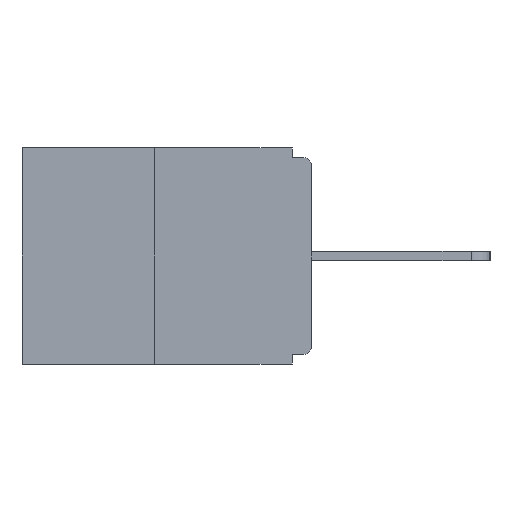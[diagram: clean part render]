
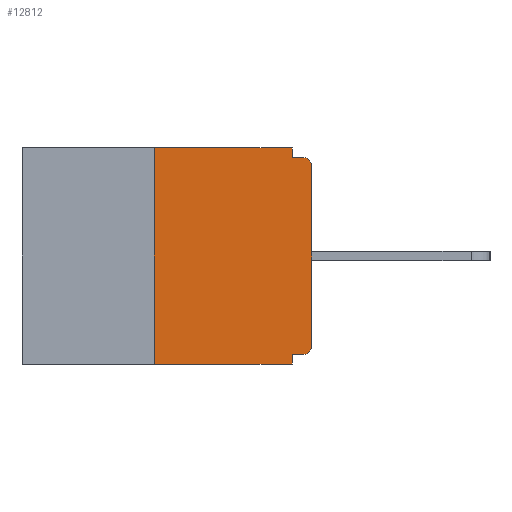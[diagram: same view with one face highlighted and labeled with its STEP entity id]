
A CAD part, left-side view. The second image highlights one B-rep face of the part: STEP entity #12812.
In plain terms, the highlighted planar face has unit normal (-1, 0, 0).
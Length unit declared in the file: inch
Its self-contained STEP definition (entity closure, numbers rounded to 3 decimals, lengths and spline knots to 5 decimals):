
#815 = CARTESIAN_POINT ( 'NONE',  ( 0., 0.015, -0.328 ) ) ;
#1198 = DIRECTION ( 'NONE',  ( 0., -1., 0. ) ) ;
#1641 = ORIENTED_EDGE ( 'NONE', *, *, #5648, .T. ) ;
#1851 = CARTESIAN_POINT ( 'NONE',  ( 0., 0.031, -0.328 ) ) ;
#2156 = CARTESIAN_POINT ( 'NONE',  ( 0., 0.25, -0.343 ) ) ;
#2439 = EDGE_LOOP ( 'NONE', ( #5505, #18324, #3972, #24910, #10209, #16772, #1641, #25115, #24776, #17463 ) ) ;
#2748 = VECTOR ( 'NONE', #23778, 39.37008 ) ;
#2814 = VERTEX_POINT ( 'NONE', #15146 ) ;
#2869 = CARTESIAN_POINT ( 'NONE',  ( 0., 0., -0.328 ) ) ;
#3316 = VECTOR ( 'NONE', #11759, 39.37008 ) ;
#3339 = DIRECTION ( 'NONE',  ( -1., 0., 0. ) ) ;
#3678 = AXIS2_PLACEMENT_3D ( 'NONE', #8820, #10789, #18756 ) ;
#3972 = ORIENTED_EDGE ( 'NONE', *, *, #20627, .T. ) ;
#4026 = CARTESIAN_POINT ( 'NONE',  ( 0., 0.015, -0.015 ) ) ;
#4176 = VERTEX_POINT ( 'NONE', #815 ) ;
#4190 = EDGE_CURVE ( 'NONE', #11388, #22368, #18947, .T. ) ;
#4318 = CIRCLE ( 'NONE', #24548, 0.015 ) ;
#4536 = CARTESIAN_POINT ( 'NONE',  ( 0., 0., -0.03 ) ) ;
#4954 = CARTESIAN_POINT ( 'NONE',  ( 0., 0.25, 0. ) ) ;
#4955 = DIRECTION ( 'NONE',  ( 0., 0., -1. ) ) ;
#5152 = EDGE_CURVE ( 'NONE', #19317, #2814, #7608, .T. ) ;
#5505 = ORIENTED_EDGE ( 'NONE', *, *, #8777, .F. ) ;
#5648 = EDGE_CURVE ( 'NONE', #12283, #21295, #25003, .T. ) ;
#5665 = CARTESIAN_POINT ( 'NONE',  ( 0., 0.25, 0. ) ) ;
#6247 = CIRCLE ( 'NONE', #14596, 0.015 ) ;
#6942 = CARTESIAN_POINT ( 'NONE',  ( 0., 0.031, 0. ) ) ;
#7402 = CARTESIAN_POINT ( 'NONE',  ( 0., 0., -0.313 ) ) ;
#7410 = FACE_OUTER_BOUND ( 'NONE', #2439, .T. ) ;
#7608 = LINE ( 'NONE', #16184, #17377 ) ;
#7834 = EDGE_CURVE ( 'NONE', #21295, #24124, #4318, .T. ) ;
#7877 = CARTESIAN_POINT ( 'NONE',  ( 0., 0., -0.015 ) ) ;
#7922 = VECTOR ( 'NONE', #10638, 39.37008 ) ;
#8051 = CARTESIAN_POINT ( 'NONE',  ( 0., 0., 0. ) ) ;
#8095 = LINE ( 'NONE', #2869, #19121 ) ;
#8693 = VECTOR ( 'NONE', #1198, 39.37008 ) ;
#8777 = EDGE_CURVE ( 'NONE', #22368, #16342, #20468, .T. ) ;
#8820 = CARTESIAN_POINT ( 'NONE',  ( 0., 0.46, 0. ) ) ;
#9101 = CARTESIAN_POINT ( 'NONE',  ( 0., 0.015, -0.03 ) ) ;
#10209 = ORIENTED_EDGE ( 'NONE', *, *, #14150, .F. ) ;
#10638 = DIRECTION ( 'NONE',  ( 0., 0., 1. ) ) ;
#10789 = DIRECTION ( 'NONE',  ( 1., 0., 0. ) ) ;
#10865 = DIRECTION ( 'NONE',  ( 0., 0., -1. ) ) ;
#11388 = VERTEX_POINT ( 'NONE', #2156 ) ;
#11759 = DIRECTION ( 'NONE',  ( 0., -1., 0. ) ) ;
#12283 = VERTEX_POINT ( 'NONE', #7402 ) ;
#12812 = ADVANCED_FACE ( 'NONE', ( #7410 ), #14660, .F. ) ;
#12859 = CARTESIAN_POINT ( 'NONE',  ( 0., 0.46, -0.343 ) ) ;
#13325 = LINE ( 'NONE', #12859, #8693 ) ;
#14150 = EDGE_CURVE ( 'NONE', #4176, #19317, #8095, .T. ) ;
#14414 = DIRECTION ( 'NONE',  ( 0., 0., -1. ) ) ;
#14596 = AXIS2_PLACEMENT_3D ( 'NONE', #22462, #16626, #4955 ) ;
#14660 = PLANE ( 'NONE',  #3678 ) ;
#14987 = VERTEX_POINT ( 'NONE', #17638 ) ;
#15146 = CARTESIAN_POINT ( 'NONE',  ( 0., 0.031, -0.343 ) ) ;
#16184 = CARTESIAN_POINT ( 'NONE',  ( 0., 0.031, -0.343 ) ) ;
#16342 = VERTEX_POINT ( 'NONE', #21648 ) ;
#16626 = DIRECTION ( 'NONE',  ( -1., 0., 0. ) ) ;
#16772 = ORIENTED_EDGE ( 'NONE', *, *, #21399, .T. ) ;
#17377 = VECTOR ( 'NONE', #14414, 39.37008 ) ;
#17463 = ORIENTED_EDGE ( 'NONE', *, *, #19082, .F. ) ;
#17638 = CARTESIAN_POINT ( 'NONE',  ( 0., 0.031, -0.015 ) ) ;
#18324 = ORIENTED_EDGE ( 'NONE', *, *, #4190, .F. ) ;
#18546 = CARTESIAN_POINT ( 'NONE',  ( 0., 0.46, 0. ) ) ;
#18629 = DIRECTION ( 'NONE',  ( 0., -1., 0. ) ) ;
#18756 = DIRECTION ( 'NONE',  ( 0., 0., -1. ) ) ;
#18947 = LINE ( 'NONE', #4954, #7922 ) ;
#19082 = EDGE_CURVE ( 'NONE', #16342, #14987, #19518, .T. ) ;
#19121 = VECTOR ( 'NONE', #20424, 39.37008 ) ;
#19194 = VECTOR ( 'NONE', #10865, 39.37008 ) ;
#19317 = VERTEX_POINT ( 'NONE', #1851 ) ;
#19518 = LINE ( 'NONE', #6942, #19194 ) ;
#20187 = VECTOR ( 'NONE', #18629, 39.37008 ) ;
#20424 = DIRECTION ( 'NONE',  ( 0., 1., 0. ) ) ;
#20468 = LINE ( 'NONE', #18546, #20187 ) ;
#20627 = EDGE_CURVE ( 'NONE', #11388, #2814, #13325, .T. ) ;
#21295 = VERTEX_POINT ( 'NONE', #4536 ) ;
#21399 = EDGE_CURVE ( 'NONE', #4176, #12283, #6247, .T. ) ;
#21648 = CARTESIAN_POINT ( 'NONE',  ( 0., 0.031, 0. ) ) ;
#22368 = VERTEX_POINT ( 'NONE', #5665 ) ;
#22462 = CARTESIAN_POINT ( 'NONE',  ( 0., 0.015, -0.313 ) ) ;
#22802 = DIRECTION ( 'NONE',  ( 0., 0., -1. ) ) ;
#23778 = DIRECTION ( 'NONE',  ( 0., 0., 1. ) ) ;
#24124 = VERTEX_POINT ( 'NONE', #4026 ) ;
#24548 = AXIS2_PLACEMENT_3D ( 'NONE', #9101, #3339, #22802 ) ;
#24624 = EDGE_CURVE ( 'NONE', #14987, #24124, #24688, .T. ) ;
#24688 = LINE ( 'NONE', #7877, #3316 ) ;
#24776 = ORIENTED_EDGE ( 'NONE', *, *, #24624, .F. ) ;
#24910 = ORIENTED_EDGE ( 'NONE', *, *, #5152, .F. ) ;
#25003 = LINE ( 'NONE', #8051, #2748 ) ;
#25115 = ORIENTED_EDGE ( 'NONE', *, *, #7834, .T. ) ;
